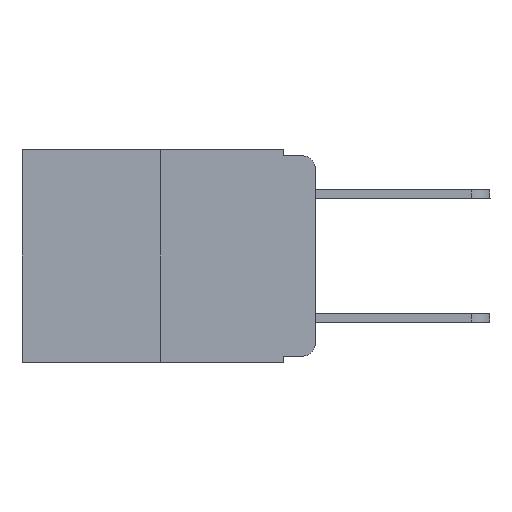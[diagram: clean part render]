
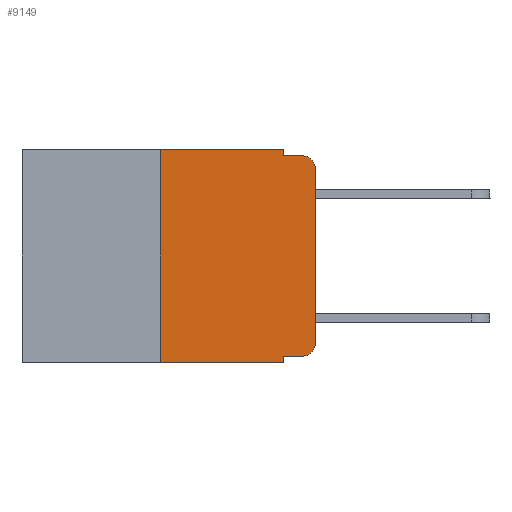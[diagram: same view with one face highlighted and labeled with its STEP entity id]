
A CAD part, left-side view. The second image highlights one B-rep face of the part: STEP entity #9149.
In plain terms, the highlighted planar face has unit normal (-1, 0, 0).
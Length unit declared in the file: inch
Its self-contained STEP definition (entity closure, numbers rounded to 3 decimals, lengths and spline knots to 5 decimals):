
#569 = LINE ( 'NONE', #17057, #22888 ) ;
#740 = CARTESIAN_POINT ( 'NONE',  ( 0., 0.473, 0. ) ) ;
#756 = VERTEX_POINT ( 'NONE', #20066 ) ;
#972 = ORIENTED_EDGE ( 'NONE', *, *, #7494, .F. ) ;
#1489 = EDGE_CURVE ( 'NONE', #21886, #756, #11817, .T. ) ;
#2067 = VECTOR ( 'NONE', #3357, 39.37008 ) ;
#2110 = EDGE_CURVE ( 'NONE', #7569, #22227, #21233, .T. ) ;
#2375 = VERTEX_POINT ( 'NONE', #11051 ) ;
#2587 = CARTESIAN_POINT ( 'NONE',  ( 0., 0.051, 0. ) ) ;
#2653 = ORIENTED_EDGE ( 'NONE', *, *, #23411, .F. ) ;
#3023 = PLANE ( 'NONE',  #13225 ) ;
#3334 = LINE ( 'NONE', #12320, #23516 ) ;
#3357 = DIRECTION ( 'NONE',  ( 0., 0., -1. ) ) ;
#3402 = LINE ( 'NONE', #8890, #23299 ) ;
#3696 = VERTEX_POINT ( 'NONE', #12983 ) ;
#3897 = DIRECTION ( 'NONE',  ( -1., 0., 0. ) ) ;
#4219 = DIRECTION ( 'NONE',  ( 0., -1., 0. ) ) ;
#4426 = CARTESIAN_POINT ( 'NONE',  ( 0., 0.051, 0. ) ) ;
#5036 = EDGE_CURVE ( 'NONE', #5519, #10714, #22507, .T. ) ;
#5209 = CARTESIAN_POINT ( 'NONE',  ( 0., 0.051, 0. ) ) ;
#5403 = VECTOR ( 'NONE', #18897, 39.37008 ) ;
#5519 = VERTEX_POINT ( 'NONE', #16046 ) ;
#7047 = CARTESIAN_POINT ( 'NONE',  ( 0., 0.473, 0. ) ) ;
#7494 = EDGE_CURVE ( 'NONE', #16087, #7569, #3402, .T. ) ;
#7569 = VERTEX_POINT ( 'NONE', #9606 ) ;
#7626 = VECTOR ( 'NONE', #17767, 39.37008 ) ;
#7663 = DIRECTION ( 'NONE',  ( 0., 0., -1. ) ) ;
#8169 = ORIENTED_EDGE ( 'NONE', *, *, #18655, .T. ) ;
#8364 = CARTESIAN_POINT ( 'NONE',  ( 0., 0., -0.313 ) ) ;
#8869 = FACE_OUTER_BOUND ( 'NONE', #10220, .T. ) ;
#8890 = CARTESIAN_POINT ( 'NONE',  ( 0., 0.25, 0. ) ) ;
#9149 = ADVANCED_FACE ( 'NONE', ( #8869 ), #3023, .F. ) ;
#9492 = AXIS2_PLACEMENT_3D ( 'NONE', #18847, #17260, #9770 ) ;
#9606 = CARTESIAN_POINT ( 'NONE',  ( 0., 0.25, 0. ) ) ;
#9770 = DIRECTION ( 'NONE',  ( 0., 0., -1. ) ) ;
#10220 = EDGE_LOOP ( 'NONE', ( #8169, #15926, #2653, #18927, #12308, #972, #14112, #15499, #22202, #21089 ) ) ;
#10427 = CARTESIAN_POINT ( 'NONE',  ( 0., 0.25, -0.343 ) ) ;
#10714 = VERTEX_POINT ( 'NONE', #8364 ) ;
#11051 = CARTESIAN_POINT ( 'NONE',  ( 0., 0.051, -0.333 ) ) ;
#11481 = LINE ( 'NONE', #4426, #13961 ) ;
#11817 = CIRCLE ( 'NONE', #9492, 0.02 ) ;
#11827 = DIRECTION ( 'NONE',  ( 0., 0., -1. ) ) ;
#11911 = DIRECTION ( 'NONE',  ( 0., -1., 0. ) ) ;
#12272 = EDGE_CURVE ( 'NONE', #2375, #3696, #21788, .T. ) ;
#12308 = ORIENTED_EDGE ( 'NONE', *, *, #2110, .F. ) ;
#12320 = CARTESIAN_POINT ( 'NONE',  ( 0., 0.051, -0.333 ) ) ;
#12785 = DIRECTION ( 'NONE',  ( 0., -1., 0. ) ) ;
#12983 = CARTESIAN_POINT ( 'NONE',  ( 0., 0.051, -0.343 ) ) ;
#13202 = CARTESIAN_POINT ( 'NONE',  ( 0., 0., 0. ) ) ;
#13225 = AXIS2_PLACEMENT_3D ( 'NONE', #7047, #23651, #14648 ) ;
#13889 = LINE ( 'NONE', #19473, #7626 ) ;
#13961 = VECTOR ( 'NONE', #11827, 39.37008 ) ;
#14112 = ORIENTED_EDGE ( 'NONE', *, *, #16414, .T. ) ;
#14606 = CARTESIAN_POINT ( 'NONE',  ( 0., 0., -0.03 ) ) ;
#14648 = DIRECTION ( 'NONE',  ( 0., 0., -1. ) ) ;
#15499 = ORIENTED_EDGE ( 'NONE', *, *, #12272, .F. ) ;
#15926 = ORIENTED_EDGE ( 'NONE', *, *, #1489, .T. ) ;
#16046 = CARTESIAN_POINT ( 'NONE',  ( 0., 0.02, -0.333 ) ) ;
#16087 = VERTEX_POINT ( 'NONE', #10427 ) ;
#16414 = EDGE_CURVE ( 'NONE', #16087, #3696, #13889, .T. ) ;
#16637 = EDGE_CURVE ( 'NONE', #2375, #5519, #3334, .T. ) ;
#17057 = CARTESIAN_POINT ( 'NONE',  ( 0., 0.051, -0.01 ) ) ;
#17260 = DIRECTION ( 'NONE',  ( -1., 0., 0. ) ) ;
#17767 = DIRECTION ( 'NONE',  ( 0., -1., 0. ) ) ;
#17871 = VERTEX_POINT ( 'NONE', #18020 ) ;
#18020 = CARTESIAN_POINT ( 'NONE',  ( 0., 0.051, -0.01 ) ) ;
#18655 = EDGE_CURVE ( 'NONE', #10714, #21886, #20614, .T. ) ;
#18847 = CARTESIAN_POINT ( 'NONE',  ( 0., 0.02, -0.03 ) ) ;
#18897 = DIRECTION ( 'NONE',  ( 0., 0., 1. ) ) ;
#18927 = ORIENTED_EDGE ( 'NONE', *, *, #22045, .F. ) ;
#19473 = CARTESIAN_POINT ( 'NONE',  ( 0., 0.473, -0.343 ) ) ;
#19974 = VECTOR ( 'NONE', #11911, 39.37008 ) ;
#20066 = CARTESIAN_POINT ( 'NONE',  ( 0., 0.02, -0.01 ) ) ;
#20614 = LINE ( 'NONE', #13202, #5403 ) ;
#21089 = ORIENTED_EDGE ( 'NONE', *, *, #5036, .T. ) ;
#21233 = LINE ( 'NONE', #740, #19974 ) ;
#21347 = AXIS2_PLACEMENT_3D ( 'NONE', #22793, #3897, #7663 ) ;
#21593 = DIRECTION ( 'NONE',  ( 0., 0., 1. ) ) ;
#21788 = LINE ( 'NONE', #5209, #2067 ) ;
#21886 = VERTEX_POINT ( 'NONE', #14606 ) ;
#22045 = EDGE_CURVE ( 'NONE', #22227, #17871, #11481, .T. ) ;
#22202 = ORIENTED_EDGE ( 'NONE', *, *, #16637, .T. ) ;
#22227 = VERTEX_POINT ( 'NONE', #2587 ) ;
#22507 = CIRCLE ( 'NONE', #21347, 0.02 ) ;
#22793 = CARTESIAN_POINT ( 'NONE',  ( 0., 0.02, -0.313 ) ) ;
#22888 = VECTOR ( 'NONE', #4219, 39.37008 ) ;
#23299 = VECTOR ( 'NONE', #21593, 39.37008 ) ;
#23411 = EDGE_CURVE ( 'NONE', #17871, #756, #569, .T. ) ;
#23516 = VECTOR ( 'NONE', #12785, 39.37008 ) ;
#23651 = DIRECTION ( 'NONE',  ( 1., 0., 0. ) ) ;
